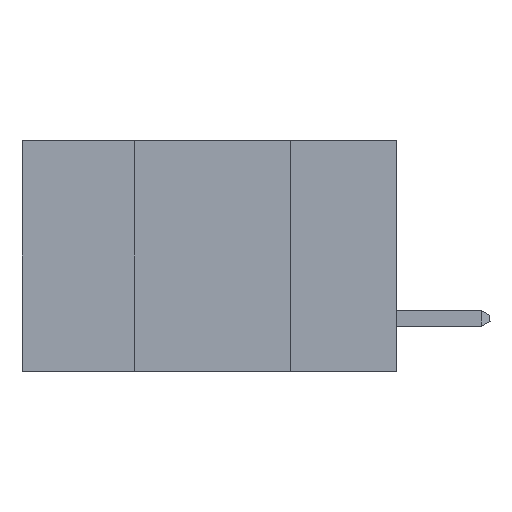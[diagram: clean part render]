
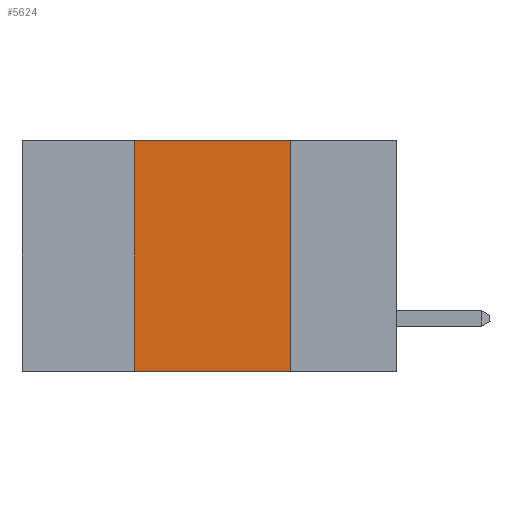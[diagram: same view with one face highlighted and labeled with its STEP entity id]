
A CAD part, left-side view. The second image highlights one B-rep face of the part: STEP entity #5624.
In plain terms, the highlighted planar face has unit normal (-1, 0, 0).
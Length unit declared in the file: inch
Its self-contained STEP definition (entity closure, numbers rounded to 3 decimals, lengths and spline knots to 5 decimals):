
#22 = PLANE ( 'NONE',  #4638 ) ;
#51 = FACE_OUTER_BOUND ( 'NONE', #5551, .T. ) ;
#577 = LINE ( 'NONE', #7441, #5405 ) ;
#1437 = DIRECTION ( 'NONE',  ( 1., 0., 0. ) ) ;
#1472 = LINE ( 'NONE', #9423, #6781 ) ;
#1784 = DIRECTION ( 'NONE',  ( 0., 0., 1. ) ) ;
#1841 = EDGE_CURVE ( 'NONE', #11334, #4146, #7738, .T. ) ;
#2378 = ORIENTED_EDGE ( 'NONE', *, *, #4472, .F. ) ;
#2904 = CARTESIAN_POINT ( 'NONE',  ( 0., 0.17, 0. ) ) ;
#3003 = VECTOR ( 'NONE', #4104, 39.37008 ) ;
#3056 = DIRECTION ( 'NONE',  ( 0., 0., -1. ) ) ;
#3087 = CARTESIAN_POINT ( 'NONE',  ( 0., 0.6, 0. ) ) ;
#3500 = DIRECTION ( 'NONE',  ( 0., -1., 0. ) ) ;
#3758 = EDGE_CURVE ( 'NONE', #4146, #7403, #10191, .T. ) ;
#4104 = DIRECTION ( 'NONE',  ( 0., 0., -1. ) ) ;
#4146 = VERTEX_POINT ( 'NONE', #2904 ) ;
#4472 = EDGE_CURVE ( 'NONE', #10588, #11334, #1472, .T. ) ;
#4638 = AXIS2_PLACEMENT_3D ( 'NONE', #11321, #1437, #3056 ) ;
#5405 = VECTOR ( 'NONE', #6527, 39.37008 ) ;
#5551 = EDGE_LOOP ( 'NONE', ( #8776, #9974, #2378, #8002 ) ) ;
#5624 = ADVANCED_FACE ( 'NONE', ( #51 ), #22, .F. ) ;
#6527 = DIRECTION ( 'NONE',  ( 0., -1., 0. ) ) ;
#6781 = VECTOR ( 'NONE', #1784, 39.37008 ) ;
#7403 = VERTEX_POINT ( 'NONE', #10767 ) ;
#7441 = CARTESIAN_POINT ( 'NONE',  ( 0., 0.6, -0.37 ) ) ;
#7738 = LINE ( 'NONE', #3087, #9745 ) ;
#7859 = CARTESIAN_POINT ( 'NONE',  ( 0., 0.17, 0. ) ) ;
#8002 = ORIENTED_EDGE ( 'NONE', *, *, #8052, .T. ) ;
#8052 = EDGE_CURVE ( 'NONE', #10588, #7403, #577, .T. ) ;
#8200 = CARTESIAN_POINT ( 'NONE',  ( 0., 0.42, -0.37 ) ) ;
#8776 = ORIENTED_EDGE ( 'NONE', *, *, #3758, .F. ) ;
#9423 = CARTESIAN_POINT ( 'NONE',  ( 0., 0.42, 0. ) ) ;
#9745 = VECTOR ( 'NONE', #3500, 39.37008 ) ;
#9974 = ORIENTED_EDGE ( 'NONE', *, *, #1841, .F. ) ;
#10191 = LINE ( 'NONE', #7859, #3003 ) ;
#10588 = VERTEX_POINT ( 'NONE', #8200 ) ;
#10611 = CARTESIAN_POINT ( 'NONE',  ( 0., 0.42, 0. ) ) ;
#10767 = CARTESIAN_POINT ( 'NONE',  ( 0., 0.17, -0.37 ) ) ;
#11321 = CARTESIAN_POINT ( 'NONE',  ( 0., 0.6, 0. ) ) ;
#11334 = VERTEX_POINT ( 'NONE', #10611 ) ;
